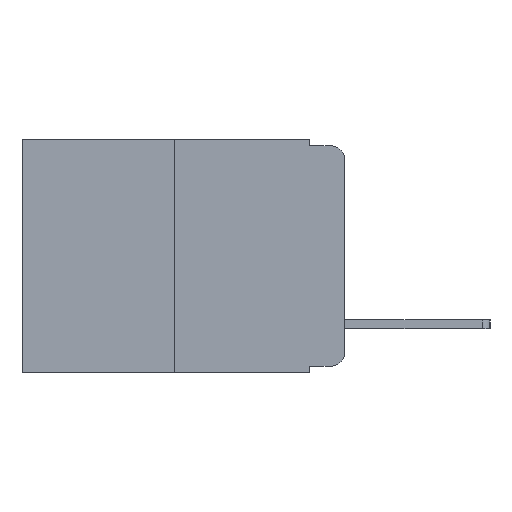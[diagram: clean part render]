
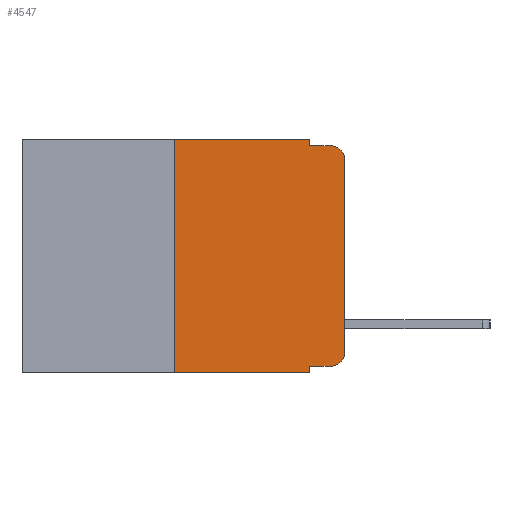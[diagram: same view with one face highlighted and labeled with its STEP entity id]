
A CAD part, left-side view. The second image highlights one B-rep face of the part: STEP entity #4547.
In plain terms, the highlighted planar face has unit normal (-1, 0, 0).
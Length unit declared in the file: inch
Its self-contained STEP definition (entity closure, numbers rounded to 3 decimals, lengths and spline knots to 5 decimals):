
#212 = CARTESIAN_POINT ( 'NONE',  ( 0., 0.473, 0. ) ) ;
#266 = ORIENTED_EDGE ( 'NONE', *, *, #2841, .F. ) ;
#282 = CARTESIAN_POINT ( 'NONE',  ( 0., 0., -0.03 ) ) ;
#328 = VERTEX_POINT ( 'NONE', #8424 ) ;
#353 = ORIENTED_EDGE ( 'NONE', *, *, #7431, .T. ) ;
#420 = VERTEX_POINT ( 'NONE', #8095 ) ;
#495 = VERTEX_POINT ( 'NONE', #7154 ) ;
#518 = DIRECTION ( 'NONE',  ( 0., 0., -1. ) ) ;
#636 = EDGE_LOOP ( 'NONE', ( #353, #661, #1142, #2800, #266, #662, #715, #860, #1377, #1964 ) ) ;
#656 = AXIS2_PLACEMENT_3D ( 'NONE', #10883, #4133, #9313 ) ;
#661 = ORIENTED_EDGE ( 'NONE', *, *, #5023, .T. ) ;
#662 = ORIENTED_EDGE ( 'NONE', *, *, #5097, .F. ) ;
#715 = ORIENTED_EDGE ( 'NONE', *, *, #1728, .T. ) ;
#845 = LINE ( 'NONE', #11165, #7860 ) ;
#860 = ORIENTED_EDGE ( 'NONE', *, *, #6970, .F. ) ;
#969 = VERTEX_POINT ( 'NONE', #10493 ) ;
#1142 = ORIENTED_EDGE ( 'NONE', *, *, #3170, .F. ) ;
#1377 = ORIENTED_EDGE ( 'NONE', *, *, #9907, .T. ) ;
#1596 = VECTOR ( 'NONE', #2509, 39.37008 ) ;
#1702 = VERTEX_POINT ( 'NONE', #2635 ) ;
#1728 = EDGE_CURVE ( 'NONE', #5790, #1702, #10376, .T. ) ;
#1758 = FACE_OUTER_BOUND ( 'NONE', #636, .T. ) ;
#1964 = ORIENTED_EDGE ( 'NONE', *, *, #7203, .T. ) ;
#2152 = VERTEX_POINT ( 'NONE', #8365 ) ;
#2206 = CARTESIAN_POINT ( 'NONE',  ( 0., 0.25, 0. ) ) ;
#2451 = CARTESIAN_POINT ( 'NONE',  ( 0., 0.02, -0.333 ) ) ;
#2509 = DIRECTION ( 'NONE',  ( 0., 0., 1. ) ) ;
#2515 = LINE ( 'NONE', #212, #9269 ) ;
#2572 = CIRCLE ( 'NONE', #4513, 0.02 ) ;
#2635 = CARTESIAN_POINT ( 'NONE',  ( 0., 0.051, -0.343 ) ) ;
#2800 = ORIENTED_EDGE ( 'NONE', *, *, #6329, .F. ) ;
#2841 = EDGE_CURVE ( 'NONE', #328, #11039, #2515, .T. ) ;
#3016 = LINE ( 'NONE', #7978, #7549 ) ;
#3170 = EDGE_CURVE ( 'NONE', #420, #495, #8613, .T. ) ;
#3986 = CARTESIAN_POINT ( 'NONE',  ( 0., 0.25, -0.343 ) ) ;
#3994 = VECTOR ( 'NONE', #6250, 39.37008 ) ;
#4071 = DIRECTION ( 'NONE',  ( 0., -1., 0. ) ) ;
#4133 = DIRECTION ( 'NONE',  ( 1., 0., 0. ) ) ;
#4231 = DIRECTION ( 'NONE',  ( 0., 0., -1. ) ) ;
#4369 = LINE ( 'NONE', #2206, #1596 ) ;
#4513 = AXIS2_PLACEMENT_3D ( 'NONE', #4935, #10790, #5858 ) ;
#4547 = ADVANCED_FACE ( 'NONE', ( #1758 ), #5047, .F. ) ;
#4589 = VERTEX_POINT ( 'NONE', #282 ) ;
#4731 = VERTEX_POINT ( 'NONE', #2451 ) ;
#4935 = CARTESIAN_POINT ( 'NONE',  ( 0., 0.02, -0.313 ) ) ;
#5023 = EDGE_CURVE ( 'NONE', #4589, #495, #9964, .T. ) ;
#5047 = PLANE ( 'NONE',  #656 ) ;
#5097 = EDGE_CURVE ( 'NONE', #5790, #328, #4369, .T. ) ;
#5479 = VECTOR ( 'NONE', #518, 39.37008 ) ;
#5790 = VERTEX_POINT ( 'NONE', #3986 ) ;
#5858 = DIRECTION ( 'NONE',  ( 0., 0., -1. ) ) ;
#5984 = VECTOR ( 'NONE', #9792, 39.37008 ) ;
#6049 = CARTESIAN_POINT ( 'NONE',  ( 0., 0.051, 0. ) ) ;
#6250 = DIRECTION ( 'NONE',  ( 0., 0., 1. ) ) ;
#6329 = EDGE_CURVE ( 'NONE', #11039, #420, #7570, .T. ) ;
#6405 = CARTESIAN_POINT ( 'NONE',  ( 0., 0.02, -0.03 ) ) ;
#6651 = DIRECTION ( 'NONE',  ( 0., 0., -1. ) ) ;
#6970 = EDGE_CURVE ( 'NONE', #969, #1702, #3016, .T. ) ;
#7154 = CARTESIAN_POINT ( 'NONE',  ( 0., 0.02, -0.01 ) ) ;
#7203 = EDGE_CURVE ( 'NONE', #4731, #2152, #2572, .T. ) ;
#7431 = EDGE_CURVE ( 'NONE', #2152, #4589, #8664, .T. ) ;
#7549 = VECTOR ( 'NONE', #4231, 39.37008 ) ;
#7570 = LINE ( 'NONE', #6049, #5479 ) ;
#7860 = VECTOR ( 'NONE', #9613, 39.37008 ) ;
#7978 = CARTESIAN_POINT ( 'NONE',  ( 0., 0.051, 0. ) ) ;
#8095 = CARTESIAN_POINT ( 'NONE',  ( 0., 0.051, -0.01 ) ) ;
#8223 = DIRECTION ( 'NONE',  ( -1., 0., 0. ) ) ;
#8365 = CARTESIAN_POINT ( 'NONE',  ( 0., 0., -0.313 ) ) ;
#8371 = VECTOR ( 'NONE', #9671, 39.37008 ) ;
#8424 = CARTESIAN_POINT ( 'NONE',  ( 0., 0.25, 0. ) ) ;
#8565 = CARTESIAN_POINT ( 'NONE',  ( 0., 0.051, -0.01 ) ) ;
#8613 = LINE ( 'NONE', #8565, #8371 ) ;
#8664 = LINE ( 'NONE', #8787, #3994 ) ;
#8695 = AXIS2_PLACEMENT_3D ( 'NONE', #6405, #8223, #6651 ) ;
#8787 = CARTESIAN_POINT ( 'NONE',  ( 0., 0., 0. ) ) ;
#9269 = VECTOR ( 'NONE', #4071, 39.37008 ) ;
#9313 = DIRECTION ( 'NONE',  ( 0., 0., -1. ) ) ;
#9613 = DIRECTION ( 'NONE',  ( 0., -1., 0. ) ) ;
#9671 = DIRECTION ( 'NONE',  ( 0., -1., 0. ) ) ;
#9792 = DIRECTION ( 'NONE',  ( 0., -1., 0. ) ) ;
#9907 = EDGE_CURVE ( 'NONE', #969, #4731, #845, .T. ) ;
#9964 = CIRCLE ( 'NONE', #8695, 0.02 ) ;
#10376 = LINE ( 'NONE', #11274, #5984 ) ;
#10493 = CARTESIAN_POINT ( 'NONE',  ( 0., 0.051, -0.333 ) ) ;
#10658 = CARTESIAN_POINT ( 'NONE',  ( 0., 0.051, 0. ) ) ;
#10790 = DIRECTION ( 'NONE',  ( -1., 0., 0. ) ) ;
#10883 = CARTESIAN_POINT ( 'NONE',  ( 0., 0.473, 0. ) ) ;
#11039 = VERTEX_POINT ( 'NONE', #10658 ) ;
#11165 = CARTESIAN_POINT ( 'NONE',  ( 0., 0.051, -0.333 ) ) ;
#11274 = CARTESIAN_POINT ( 'NONE',  ( 0., 0.473, -0.343 ) ) ;
